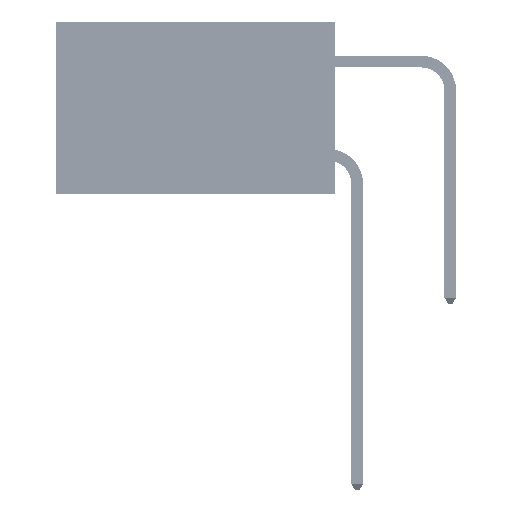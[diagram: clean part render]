
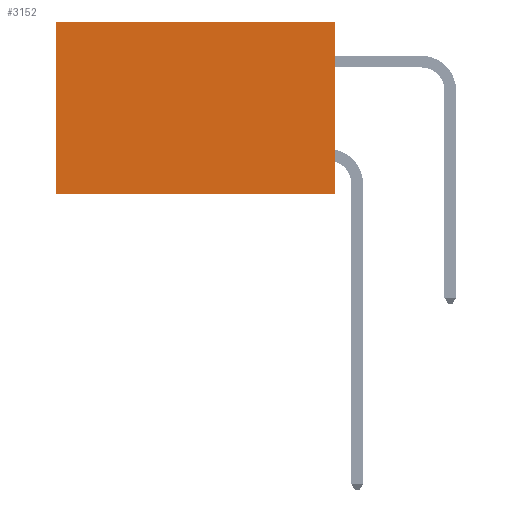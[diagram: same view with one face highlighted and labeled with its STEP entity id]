
A CAD part, left-side view. The second image highlights one B-rep face of the part: STEP entity #3152.
In plain terms, the highlighted planar face has unit normal (-1, 0, 0).
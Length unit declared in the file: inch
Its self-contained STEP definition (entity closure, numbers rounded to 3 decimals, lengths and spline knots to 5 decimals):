
#910 = LINE ( 'NONE', #19996, #22108 ) ;
#1235 = VERTEX_POINT ( 'NONE', #7402 ) ;
#2041 = VERTEX_POINT ( 'NONE', #30772 ) ;
#2742 = ORIENTED_EDGE ( 'NONE', *, *, #17513, .F. ) ;
#3152 = ADVANCED_FACE ( 'NONE', ( #44416 ), #41533, .F. ) ;
#3242 = EDGE_CURVE ( 'NONE', #1235, #2041, #910, .T. ) ;
#3818 = LINE ( 'NONE', #40964, #18495 ) ;
#4903 = DIRECTION ( 'NONE',  ( 0., 1., 0. ) ) ;
#5062 = ORIENTED_EDGE ( 'NONE', *, *, #27158, .T. ) ;
#7402 = CARTESIAN_POINT ( 'NONE',  ( 0.2875, 0., 0. ) ) ;
#8005 = DIRECTION ( 'NONE',  ( 0., 0., -1. ) ) ;
#11905 = VERTEX_POINT ( 'NONE', #44765 ) ;
#12815 = VECTOR ( 'NONE', #47774, 39.37008 ) ;
#16301 = AXIS2_PLACEMENT_3D ( 'NONE', #37718, #19670, #8005 ) ;
#17513 = EDGE_CURVE ( 'NONE', #2041, #11905, #33563, .T. ) ;
#17538 = CARTESIAN_POINT ( 'NONE',  ( 0.2875, 0.6, 0. ) ) ;
#18337 = VERTEX_POINT ( 'NONE', #17538 ) ;
#18495 = VECTOR ( 'NONE', #41445, 39.37008 ) ;
#19122 = EDGE_LOOP ( 'NONE', ( #5062, #2742, #36608, #23788 ) ) ;
#19670 = DIRECTION ( 'NONE',  ( 1., 0., 0. ) ) ;
#19996 = CARTESIAN_POINT ( 'NONE',  ( 0.2875, 0., 0. ) ) ;
#22108 = VECTOR ( 'NONE', #31267, 39.37008 ) ;
#23788 = ORIENTED_EDGE ( 'NONE', *, *, #33215, .T. ) ;
#27158 = EDGE_CURVE ( 'NONE', #18337, #11905, #3818, .T. ) ;
#30772 = CARTESIAN_POINT ( 'NONE',  ( 0.2875, 0., -0.37 ) ) ;
#30949 = CARTESIAN_POINT ( 'NONE',  ( 0.2875, 0., -0.37 ) ) ;
#31267 = DIRECTION ( 'NONE',  ( 0., 0., -1. ) ) ;
#33215 = EDGE_CURVE ( 'NONE', #1235, #18337, #41155, .T. ) ;
#33563 = LINE ( 'NONE', #30949, #42435 ) ;
#35272 = CARTESIAN_POINT ( 'NONE',  ( 0.2875, 0., 0. ) ) ;
#36608 = ORIENTED_EDGE ( 'NONE', *, *, #3242, .F. ) ;
#37718 = CARTESIAN_POINT ( 'NONE',  ( 0.2875, 0., 0. ) ) ;
#40964 = CARTESIAN_POINT ( 'NONE',  ( 0.2875, 0.6, 0. ) ) ;
#41155 = LINE ( 'NONE', #35272, #12815 ) ;
#41445 = DIRECTION ( 'NONE',  ( 0., 0., -1. ) ) ;
#41533 = PLANE ( 'NONE',  #16301 ) ;
#42435 = VECTOR ( 'NONE', #4903, 39.37008 ) ;
#44416 = FACE_OUTER_BOUND ( 'NONE', #19122, .T. ) ;
#44765 = CARTESIAN_POINT ( 'NONE',  ( 0.2875, 0.6, -0.37 ) ) ;
#47774 = DIRECTION ( 'NONE',  ( 0., 1., 0. ) ) ;
